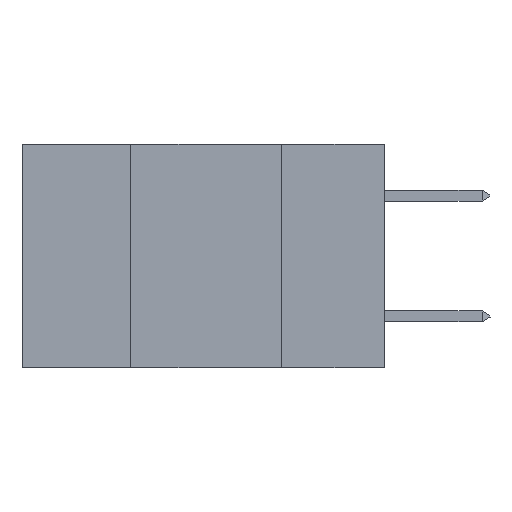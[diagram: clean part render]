
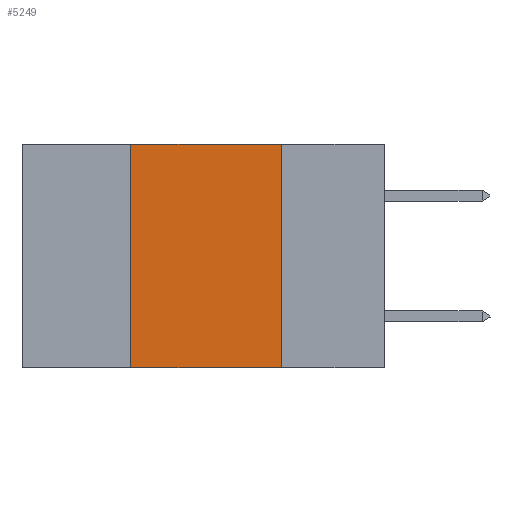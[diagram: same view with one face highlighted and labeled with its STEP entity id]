
A CAD part, left-side view. The second image highlights one B-rep face of the part: STEP entity #5249.
In plain terms, the highlighted planar face has unit normal (-1, 0, 0).
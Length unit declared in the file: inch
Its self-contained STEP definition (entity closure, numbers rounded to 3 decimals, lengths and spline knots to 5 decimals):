
#1150 = ORIENTED_EDGE ( 'NONE', *, *, #2107, .F. ) ;
#2013 = VERTEX_POINT ( 'NONE', #5257 ) ;
#2107 = EDGE_CURVE ( 'NONE', #19376, #2451, #12227, .T. ) ;
#2451 = VERTEX_POINT ( 'NONE', #19732 ) ;
#2698 = AXIS2_PLACEMENT_3D ( 'NONE', #25020, #18896, #20812 ) ;
#2822 = VECTOR ( 'NONE', #21058, 39.37008 ) ;
#3376 = DIRECTION ( 'NONE',  ( 0., 0., 1. ) ) ;
#3783 = FACE_OUTER_BOUND ( 'NONE', #10134, .T. ) ;
#4997 = EDGE_CURVE ( 'NONE', #2451, #16089, #21899, .T. ) ;
#5249 = ADVANCED_FACE ( 'NONE', ( #3783 ), #6417, .F. ) ;
#5257 = CARTESIAN_POINT ( 'NONE',  ( 0., 0.17, -0.37 ) ) ;
#6417 = PLANE ( 'NONE',  #2698 ) ;
#8357 = CARTESIAN_POINT ( 'NONE',  ( 0., 0.17, 0. ) ) ;
#8654 = LINE ( 'NONE', #8357, #11907 ) ;
#10134 = EDGE_LOOP ( 'NONE', ( #22753, #15887, #1150, #13085 ) ) ;
#11179 = CARTESIAN_POINT ( 'NONE',  ( 0., 0.6, -0.37 ) ) ;
#11907 = VECTOR ( 'NONE', #22514, 39.37008 ) ;
#12227 = LINE ( 'NONE', #26185, #22906 ) ;
#12308 = EDGE_CURVE ( 'NONE', #16089, #2013, #8654, .T. ) ;
#13085 = ORIENTED_EDGE ( 'NONE', *, *, #14956, .T. ) ;
#13806 = CARTESIAN_POINT ( 'NONE',  ( 0., 0.42, -0.37 ) ) ;
#14072 = DIRECTION ( 'NONE',  ( 0., -1., 0. ) ) ;
#14956 = EDGE_CURVE ( 'NONE', #19376, #2013, #26013, .T. ) ;
#15887 = ORIENTED_EDGE ( 'NONE', *, *, #4997, .F. ) ;
#16089 = VERTEX_POINT ( 'NONE', #21785 ) ;
#18306 = VECTOR ( 'NONE', #14072, 39.37008 ) ;
#18896 = DIRECTION ( 'NONE',  ( 1., 0., 0. ) ) ;
#19376 = VERTEX_POINT ( 'NONE', #13806 ) ;
#19732 = CARTESIAN_POINT ( 'NONE',  ( 0., 0.42, 0. ) ) ;
#20812 = DIRECTION ( 'NONE',  ( 0., 0., -1. ) ) ;
#21058 = DIRECTION ( 'NONE',  ( 0., -1., 0. ) ) ;
#21785 = CARTESIAN_POINT ( 'NONE',  ( 0., 0.17, 0. ) ) ;
#21899 = LINE ( 'NONE', #25708, #2822 ) ;
#22514 = DIRECTION ( 'NONE',  ( 0., 0., -1. ) ) ;
#22753 = ORIENTED_EDGE ( 'NONE', *, *, #12308, .F. ) ;
#22906 = VECTOR ( 'NONE', #3376, 39.37008 ) ;
#25020 = CARTESIAN_POINT ( 'NONE',  ( 0., 0.6, 0. ) ) ;
#25708 = CARTESIAN_POINT ( 'NONE',  ( 0., 0.6, 0. ) ) ;
#26013 = LINE ( 'NONE', #11179, #18306 ) ;
#26185 = CARTESIAN_POINT ( 'NONE',  ( 0., 0.42, 0. ) ) ;
